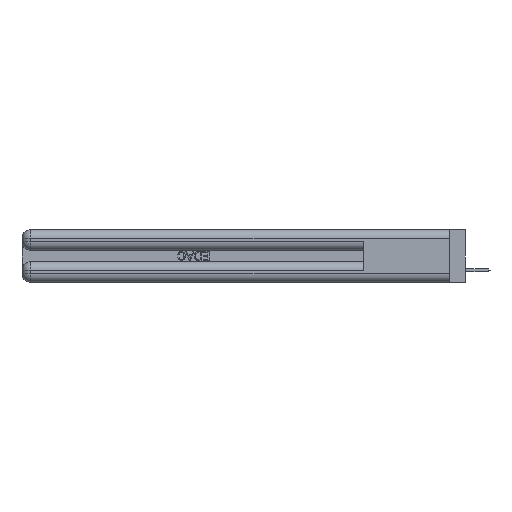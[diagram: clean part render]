
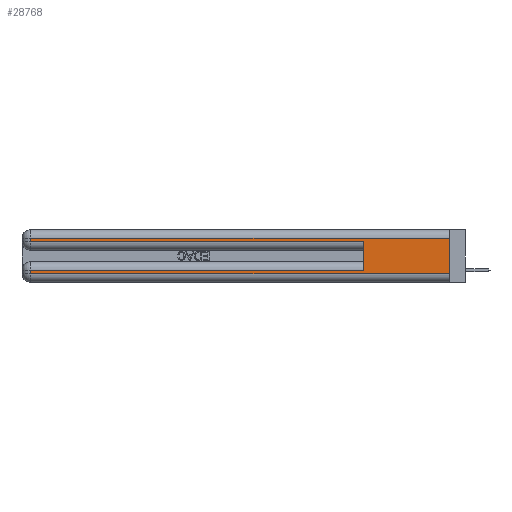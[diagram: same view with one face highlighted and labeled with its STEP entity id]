
A CAD part, left-side view. The second image highlights one B-rep face of the part: STEP entity #28768.
In plain terms, the highlighted planar face has unit normal (-1, 0, 0).
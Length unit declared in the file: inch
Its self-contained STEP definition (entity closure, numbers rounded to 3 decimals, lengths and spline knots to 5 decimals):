
#411 = LINE ( 'NONE', #8096, #34392 ) ;
#810 = DIRECTION ( 'NONE',  ( 1., 0., 0. ) ) ;
#1168 = ORIENTED_EDGE ( 'NONE', *, *, #39875, .T. ) ;
#2082 = ORIENTED_EDGE ( 'NONE', *, *, #24412, .F. ) ;
#2255 = FACE_OUTER_BOUND ( 'NONE', #17560, .T. ) ;
#3000 = DIRECTION ( 'NONE',  ( 0., -1., 0. ) ) ;
#3190 = VECTOR ( 'NONE', #17299, 39.37008 ) ;
#5139 = VECTOR ( 'NONE', #13723, 39.37008 ) ;
#5147 = EDGE_CURVE ( 'NONE', #13517, #10144, #6573, .T. ) ;
#5253 = LINE ( 'NONE', #40541, #37718 ) ;
#5318 = VERTEX_POINT ( 'NONE', #23945 ) ;
#6573 = LINE ( 'NONE', #19154, #3190 ) ;
#7197 = CARTESIAN_POINT ( 'NONE',  ( 0., 0., 0.37 ) ) ;
#7355 = ORIENTED_EDGE ( 'NONE', *, *, #26741, .F. ) ;
#7744 = LINE ( 'NONE', #39030, #23440 ) ;
#7783 = VERTEX_POINT ( 'NONE', #21404 ) ;
#8096 = CARTESIAN_POINT ( 'NONE',  ( 0., 2.94, 0.37 ) ) ;
#8128 = DIRECTION ( 'NONE',  ( 0., 1., 0. ) ) ;
#10144 = VERTEX_POINT ( 'NONE', #17216 ) ;
#13517 = VERTEX_POINT ( 'NONE', #19775 ) ;
#13723 = DIRECTION ( 'NONE',  ( 0., 1., 0. ) ) ;
#14880 = EDGE_CURVE ( 'NONE', #17852, #5318, #36635, .T. ) ;
#15275 = VERTEX_POINT ( 'NONE', #21207 ) ;
#15783 = ORIENTED_EDGE ( 'NONE', *, *, #14880, .T. ) ;
#16355 = CARTESIAN_POINT ( 'NONE',  ( 0., 2.94, 0.06 ) ) ;
#17031 = CARTESIAN_POINT ( 'NONE',  ( 0., 0., 0.31 ) ) ;
#17216 = CARTESIAN_POINT ( 'NONE',  ( 0., 0.6, 0.285 ) ) ;
#17299 = DIRECTION ( 'NONE',  ( 0., -1., 0. ) ) ;
#17560 = EDGE_LOOP ( 'NONE', ( #2082, #15783, #1168, #21940, #7355, #21197, #33053, #35987 ) ) ;
#17580 = CARTESIAN_POINT ( 'NONE',  ( 0., 0.6, 0.085 ) ) ;
#17852 = VERTEX_POINT ( 'NONE', #18764 ) ;
#18388 = EDGE_CURVE ( 'NONE', #15275, #37139, #411, .T. ) ;
#18764 = CARTESIAN_POINT ( 'NONE',  ( 0., 0., 0.31 ) ) ;
#19154 = CARTESIAN_POINT ( 'NONE',  ( 0., 0., 0.285 ) ) ;
#19775 = CARTESIAN_POINT ( 'NONE',  ( 0., 2.94, 0.285 ) ) ;
#21197 = ORIENTED_EDGE ( 'NONE', *, *, #33173, .T. ) ;
#21207 = CARTESIAN_POINT ( 'NONE',  ( 0., 2.94, 0.085 ) ) ;
#21404 = CARTESIAN_POINT ( 'NONE',  ( 0., 0., 0.06 ) ) ;
#21940 = ORIENTED_EDGE ( 'NONE', *, *, #5147, .T. ) ;
#22562 = LINE ( 'NONE', #29887, #36400 ) ;
#22729 = VERTEX_POINT ( 'NONE', #17580 ) ;
#23440 = VECTOR ( 'NONE', #8128, 39.37008 ) ;
#23945 = CARTESIAN_POINT ( 'NONE',  ( 0., 2.94, 0.31 ) ) ;
#24412 = EDGE_CURVE ( 'NONE', #17852, #7783, #38531, .T. ) ;
#25836 = DIRECTION ( 'NONE',  ( 0., 0., -1. ) ) ;
#25971 = PLANE ( 'NONE',  #29422 ) ;
#26741 = EDGE_CURVE ( 'NONE', #22729, #10144, #38828, .T. ) ;
#27556 = DIRECTION ( 'NONE',  ( 0., 0., -1. ) ) ;
#28661 = DIRECTION ( 'NONE',  ( 0., 0., -1. ) ) ;
#28768 = ADVANCED_FACE ( 'NONE', ( #2255 ), #25971, .F. ) ;
#28890 = CARTESIAN_POINT ( 'NONE',  ( 0., 0., 0.37 ) ) ;
#29000 = CARTESIAN_POINT ( 'NONE',  ( 0., 0.6, 0.145 ) ) ;
#29422 = AXIS2_PLACEMENT_3D ( 'NONE', #28890, #810, #25836 ) ;
#29694 = VECTOR ( 'NONE', #27556, 39.37008 ) ;
#29887 = CARTESIAN_POINT ( 'NONE',  ( 0., 2.94, 0.37 ) ) ;
#33049 = DIRECTION ( 'NONE',  ( 0., 0., -1. ) ) ;
#33053 = ORIENTED_EDGE ( 'NONE', *, *, #18388, .T. ) ;
#33153 = DIRECTION ( 'NONE',  ( 0., 0., 1. ) ) ;
#33173 = EDGE_CURVE ( 'NONE', #22729, #15275, #7744, .T. ) ;
#33460 = EDGE_CURVE ( 'NONE', #37139, #7783, #5253, .T. ) ;
#34392 = VECTOR ( 'NONE', #28661, 39.37008 ) ;
#35987 = ORIENTED_EDGE ( 'NONE', *, *, #33460, .T. ) ;
#36400 = VECTOR ( 'NONE', #33049, 39.37008 ) ;
#36635 = LINE ( 'NONE', #17031, #5139 ) ;
#37139 = VERTEX_POINT ( 'NONE', #16355 ) ;
#37718 = VECTOR ( 'NONE', #3000, 39.37008 ) ;
#38531 = LINE ( 'NONE', #7197, #29694 ) ;
#38828 = LINE ( 'NONE', #29000, #39340 ) ;
#39030 = CARTESIAN_POINT ( 'NONE',  ( 0., 0., 0.085 ) ) ;
#39340 = VECTOR ( 'NONE', #33153, 39.37008 ) ;
#39875 = EDGE_CURVE ( 'NONE', #5318, #13517, #22562, .T. ) ;
#40541 = CARTESIAN_POINT ( 'NONE',  ( 0., 0., 0.06 ) ) ;
